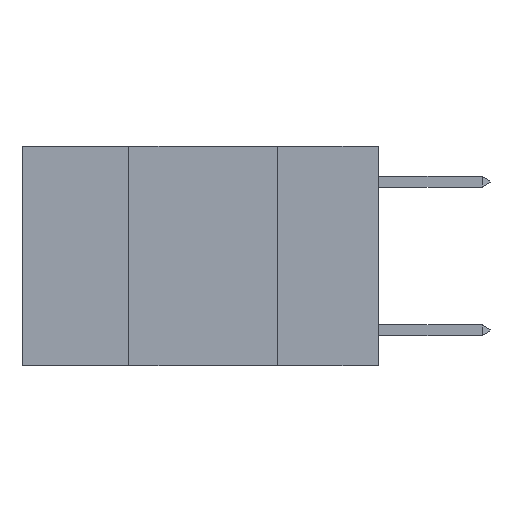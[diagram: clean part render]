
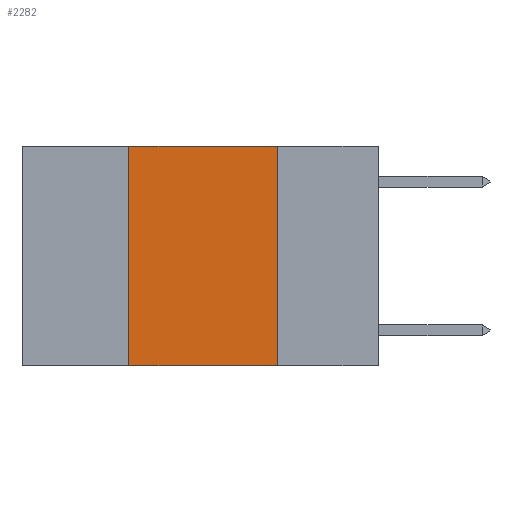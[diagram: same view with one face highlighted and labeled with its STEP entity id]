
A CAD part, left-side view. The second image highlights one B-rep face of the part: STEP entity #2282.
In plain terms, the highlighted planar face has unit normal (-1, 0, 0).
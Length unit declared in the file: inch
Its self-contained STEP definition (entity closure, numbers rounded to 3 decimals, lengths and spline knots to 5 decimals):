
#696 = LINE ( 'NONE', #20121, #3554 ) ;
#1568 = LINE ( 'NONE', #4976, #3592 ) ;
#2282 = ADVANCED_FACE ( 'NONE', ( #10599 ), #17043, .F. ) ;
#3130 = CARTESIAN_POINT ( 'NONE',  ( 0., 0.6, 0. ) ) ;
#3554 = VECTOR ( 'NONE', #20026, 39.37008 ) ;
#3592 = VECTOR ( 'NONE', #12725, 39.37008 ) ;
#4413 = VECTOR ( 'NONE', #7637, 39.37008 ) ;
#4630 = VERTEX_POINT ( 'NONE', #20890 ) ;
#4693 = DIRECTION ( 'NONE',  ( 0., 0., -1. ) ) ;
#4976 = CARTESIAN_POINT ( 'NONE',  ( 0., 0.6, 0. ) ) ;
#4977 = EDGE_CURVE ( 'NONE', #4630, #13821, #1568, .T. ) ;
#6643 = DIRECTION ( 'NONE',  ( 1., 0., 0. ) ) ;
#6652 = EDGE_CURVE ( 'NONE', #13821, #6709, #18741, .T. ) ;
#6709 = VERTEX_POINT ( 'NONE', #13977 ) ;
#7294 = CARTESIAN_POINT ( 'NONE',  ( 0., 0.17, 0. ) ) ;
#7637 = DIRECTION ( 'NONE',  ( 0., -1., 0. ) ) ;
#8349 = EDGE_CURVE ( 'NONE', #20059, #4630, #696, .T. ) ;
#8511 = EDGE_LOOP ( 'NONE', ( #15596, #13705, #20388, #11680 ) ) ;
#9314 = DIRECTION ( 'NONE',  ( 0., 0., -1. ) ) ;
#10599 = FACE_OUTER_BOUND ( 'NONE', #8511, .T. ) ;
#11680 = ORIENTED_EDGE ( 'NONE', *, *, #16399, .T. ) ;
#12725 = DIRECTION ( 'NONE',  ( 0., -1., 0. ) ) ;
#13705 = ORIENTED_EDGE ( 'NONE', *, *, #4977, .F. ) ;
#13818 = CARTESIAN_POINT ( 'NONE',  ( 0., 0.17, 0. ) ) ;
#13821 = VERTEX_POINT ( 'NONE', #13818 ) ;
#13977 = CARTESIAN_POINT ( 'NONE',  ( 0., 0.17, -0.37 ) ) ;
#14393 = CARTESIAN_POINT ( 'NONE',  ( 0., 0.6, -0.37 ) ) ;
#15596 = ORIENTED_EDGE ( 'NONE', *, *, #6652, .F. ) ;
#15769 = VECTOR ( 'NONE', #9314, 39.37008 ) ;
#16399 = EDGE_CURVE ( 'NONE', #20059, #6709, #17259, .T. ) ;
#17043 = PLANE ( 'NONE',  #19896 ) ;
#17259 = LINE ( 'NONE', #14393, #4413 ) ;
#18741 = LINE ( 'NONE', #7294, #15769 ) ;
#19896 = AXIS2_PLACEMENT_3D ( 'NONE', #3130, #6643, #4693 ) ;
#20026 = DIRECTION ( 'NONE',  ( 0., 0., 1. ) ) ;
#20059 = VERTEX_POINT ( 'NONE', #20711 ) ;
#20121 = CARTESIAN_POINT ( 'NONE',  ( 0., 0.42, 0. ) ) ;
#20388 = ORIENTED_EDGE ( 'NONE', *, *, #8349, .F. ) ;
#20711 = CARTESIAN_POINT ( 'NONE',  ( 0., 0.42, -0.37 ) ) ;
#20890 = CARTESIAN_POINT ( 'NONE',  ( 0., 0.42, 0. ) ) ;
